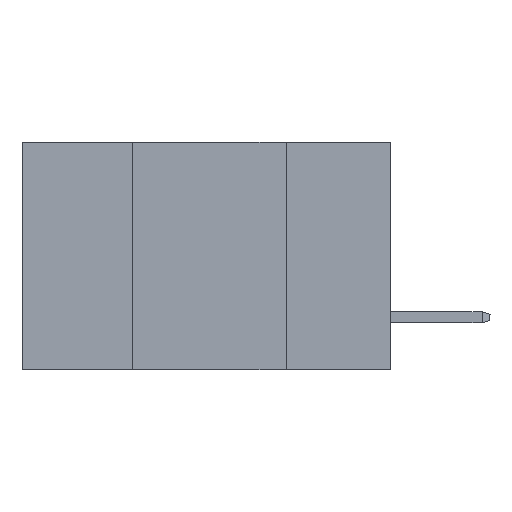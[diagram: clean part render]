
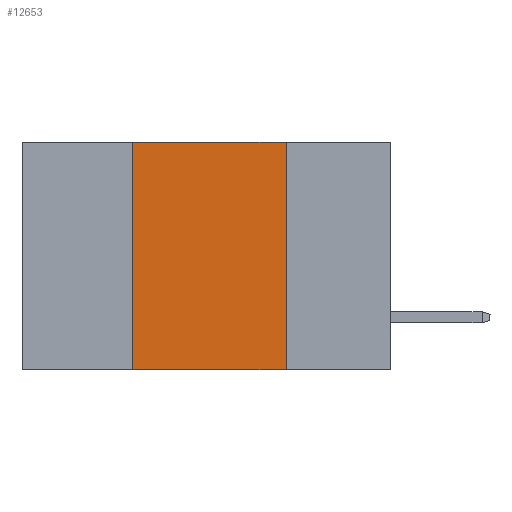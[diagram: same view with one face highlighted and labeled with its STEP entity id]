
A CAD part, left-side view. The second image highlights one B-rep face of the part: STEP entity #12653.
In plain terms, the highlighted planar face has unit normal (-1, 0, 0).
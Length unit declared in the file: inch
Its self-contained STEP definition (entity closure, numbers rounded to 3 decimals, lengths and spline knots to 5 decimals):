
#606 = EDGE_LOOP ( 'NONE', ( #3947, #13593, #16150, #9539 ) ) ;
#764 = DIRECTION ( 'NONE',  ( 0., -1., 0. ) ) ;
#2672 = EDGE_CURVE ( 'NONE', #20670, #4539, #5316, .T. ) ;
#3855 = CARTESIAN_POINT ( 'NONE',  ( 0., 0.6, 0. ) ) ;
#3947 = ORIENTED_EDGE ( 'NONE', *, *, #8162, .F. ) ;
#4145 = CARTESIAN_POINT ( 'NONE',  ( 0., 0.6, -0.37 ) ) ;
#4174 = LINE ( 'NONE', #16082, #7832 ) ;
#4398 = DIRECTION ( 'NONE',  ( 0., 0., 1. ) ) ;
#4539 = VERTEX_POINT ( 'NONE', #13690 ) ;
#5316 = LINE ( 'NONE', #18674, #6447 ) ;
#6447 = VECTOR ( 'NONE', #4398, 39.37008 ) ;
#7273 = EDGE_CURVE ( 'NONE', #4539, #8502, #4174, .T. ) ;
#7406 = PLANE ( 'NONE',  #11189 ) ;
#7758 = VECTOR ( 'NONE', #764, 39.37008 ) ;
#7832 = VECTOR ( 'NONE', #16243, 39.37008 ) ;
#8162 = EDGE_CURVE ( 'NONE', #8502, #16735, #20380, .T. ) ;
#8502 = VERTEX_POINT ( 'NONE', #10277 ) ;
#9539 = ORIENTED_EDGE ( 'NONE', *, *, #22984, .T. ) ;
#10277 = CARTESIAN_POINT ( 'NONE',  ( 0., 0.17, 0. ) ) ;
#11189 = AXIS2_PLACEMENT_3D ( 'NONE', #3855, #18139, #16140 ) ;
#11744 = FACE_OUTER_BOUND ( 'NONE', #606, .T. ) ;
#12653 = ADVANCED_FACE ( 'NONE', ( #11744 ), #7406, .F. ) ;
#13593 = ORIENTED_EDGE ( 'NONE', *, *, #7273, .F. ) ;
#13634 = VECTOR ( 'NONE', #17672, 39.37008 ) ;
#13690 = CARTESIAN_POINT ( 'NONE',  ( 0., 0.42, 0. ) ) ;
#15815 = CARTESIAN_POINT ( 'NONE',  ( 0., 0.17, 0. ) ) ;
#16082 = CARTESIAN_POINT ( 'NONE',  ( 0., 0.6, 0. ) ) ;
#16140 = DIRECTION ( 'NONE',  ( 0., 0., -1. ) ) ;
#16150 = ORIENTED_EDGE ( 'NONE', *, *, #2672, .F. ) ;
#16243 = DIRECTION ( 'NONE',  ( 0., -1., 0. ) ) ;
#16735 = VERTEX_POINT ( 'NONE', #19196 ) ;
#17672 = DIRECTION ( 'NONE',  ( 0., 0., -1. ) ) ;
#18139 = DIRECTION ( 'NONE',  ( 1., 0., 0. ) ) ;
#18674 = CARTESIAN_POINT ( 'NONE',  ( 0., 0.42, 0. ) ) ;
#19196 = CARTESIAN_POINT ( 'NONE',  ( 0., 0.17, -0.37 ) ) ;
#20380 = LINE ( 'NONE', #15815, #13634 ) ;
#20670 = VERTEX_POINT ( 'NONE', #20785 ) ;
#20785 = CARTESIAN_POINT ( 'NONE',  ( 0., 0.42, -0.37 ) ) ;
#20920 = LINE ( 'NONE', #4145, #7758 ) ;
#22984 = EDGE_CURVE ( 'NONE', #20670, #16735, #20920, .T. ) ;
